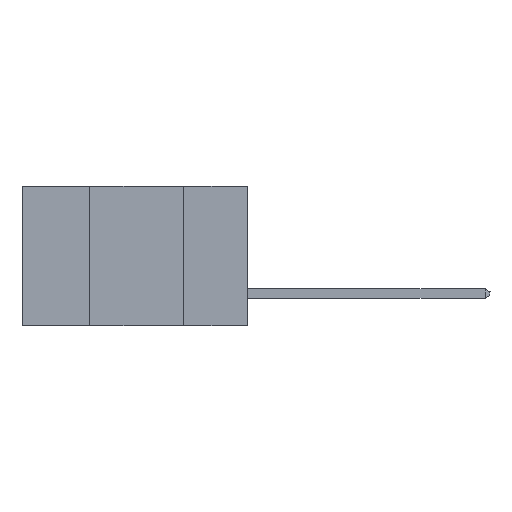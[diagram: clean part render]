
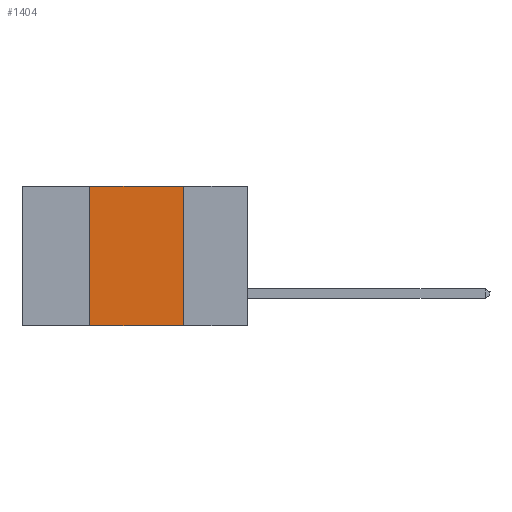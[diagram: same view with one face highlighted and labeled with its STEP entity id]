
A CAD part, left-side view. The second image highlights one B-rep face of the part: STEP entity #1404.
In plain terms, the highlighted planar face has unit normal (-1, 0, 0).
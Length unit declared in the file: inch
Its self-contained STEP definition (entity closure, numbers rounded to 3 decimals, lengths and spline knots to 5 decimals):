
#282 = VECTOR ( 'NONE', #16113, 39.37008 ) ;
#805 = CARTESIAN_POINT ( 'NONE',  ( 0., 0.17, 0. ) ) ;
#1198 = DIRECTION ( 'NONE',  ( 1., 0., 0. ) ) ;
#1404 = ADVANCED_FACE ( 'NONE', ( #16896 ), #7789, .F. ) ;
#1998 = VERTEX_POINT ( 'NONE', #6792 ) ;
#2271 = VECTOR ( 'NONE', #15712, 39.37008 ) ;
#3011 = CARTESIAN_POINT ( 'NONE',  ( 0., 0.42, -0.37 ) ) ;
#3655 = VECTOR ( 'NONE', #10150, 39.37008 ) ;
#4766 = EDGE_LOOP ( 'NONE', ( #11000, #17030, #5202, #5471 ) ) ;
#4950 = LINE ( 'NONE', #12980, #11167 ) ;
#5202 = ORIENTED_EDGE ( 'NONE', *, *, #14586, .F. ) ;
#5471 = ORIENTED_EDGE ( 'NONE', *, *, #11910, .T. ) ;
#5942 = EDGE_CURVE ( 'NONE', #1998, #11423, #4950, .T. ) ;
#6505 = DIRECTION ( 'NONE',  ( 0., 0., -1. ) ) ;
#6792 = CARTESIAN_POINT ( 'NONE',  ( 0., 0.42, 0. ) ) ;
#7789 = PLANE ( 'NONE',  #10770 ) ;
#8079 = CARTESIAN_POINT ( 'NONE',  ( 0., 0.6, -0.37 ) ) ;
#8302 = LINE ( 'NONE', #3011, #282 ) ;
#8616 = EDGE_CURVE ( 'NONE', #11423, #11561, #16924, .T. ) ;
#10150 = DIRECTION ( 'NONE',  ( 0., 0., -1. ) ) ;
#10770 = AXIS2_PLACEMENT_3D ( 'NONE', #13042, #1198, #6505 ) ;
#11000 = ORIENTED_EDGE ( 'NONE', *, *, #8616, .F. ) ;
#11167 = VECTOR ( 'NONE', #15698, 39.37008 ) ;
#11423 = VERTEX_POINT ( 'NONE', #805 ) ;
#11538 = VERTEX_POINT ( 'NONE', #14742 ) ;
#11561 = VERTEX_POINT ( 'NONE', #13447 ) ;
#11910 = EDGE_CURVE ( 'NONE', #11538, #11561, #12267, .T. ) ;
#12267 = LINE ( 'NONE', #8079, #2271 ) ;
#12980 = CARTESIAN_POINT ( 'NONE',  ( 0., 0.6, 0. ) ) ;
#13042 = CARTESIAN_POINT ( 'NONE',  ( 0., 0.6, 0. ) ) ;
#13447 = CARTESIAN_POINT ( 'NONE',  ( 0., 0.17, -0.37 ) ) ;
#14295 = CARTESIAN_POINT ( 'NONE',  ( 0., 0.17, -0.37 ) ) ;
#14586 = EDGE_CURVE ( 'NONE', #11538, #1998, #8302, .T. ) ;
#14742 = CARTESIAN_POINT ( 'NONE',  ( 0., 0.42, -0.37 ) ) ;
#15698 = DIRECTION ( 'NONE',  ( 0., -1., 0. ) ) ;
#15712 = DIRECTION ( 'NONE',  ( 0., -1., 0. ) ) ;
#16113 = DIRECTION ( 'NONE',  ( 0., 0., 1. ) ) ;
#16896 = FACE_OUTER_BOUND ( 'NONE', #4766, .T. ) ;
#16924 = LINE ( 'NONE', #14295, #3655 ) ;
#17030 = ORIENTED_EDGE ( 'NONE', *, *, #5942, .F. ) ;
